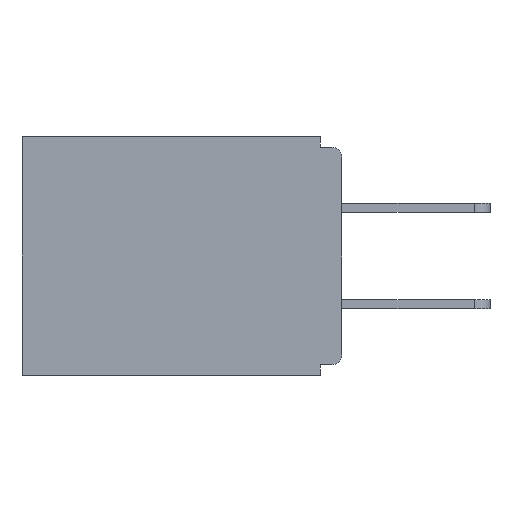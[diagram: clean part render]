
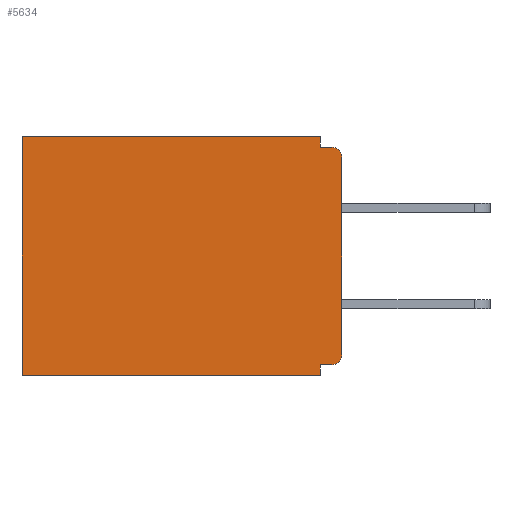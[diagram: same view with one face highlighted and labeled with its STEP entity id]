
A CAD part, left-side view. The second image highlights one B-rep face of the part: STEP entity #5634.
In plain terms, the highlighted planar face has unit normal (-1, 0, 0).
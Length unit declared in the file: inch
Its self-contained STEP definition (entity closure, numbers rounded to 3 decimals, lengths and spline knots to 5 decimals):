
#144 = VERTEX_POINT ( 'NONE', #15866 ) ;
#298 = VECTOR ( 'NONE', #16780, 39.37008 ) ;
#392 = DIRECTION ( 'NONE',  ( 0., 0., -1. ) ) ;
#428 = EDGE_CURVE ( 'NONE', #17263, #8227, #17666, .T. ) ;
#733 = ORIENTED_EDGE ( 'NONE', *, *, #4994, .F. ) ;
#946 = VECTOR ( 'NONE', #20086, 39.37008 ) ;
#1278 = CARTESIAN_POINT ( 'NONE',  ( 0.298, 0., -0.343 ) ) ;
#1414 = DIRECTION ( 'NONE',  ( -1., 0., 0. ) ) ;
#1761 = EDGE_CURVE ( 'NONE', #11068, #144, #8837, .T. ) ;
#1814 = VERTEX_POINT ( 'NONE', #16968 ) ;
#1829 = PLANE ( 'NONE',  #11761 ) ;
#2190 = DIRECTION ( 'NONE',  ( 0., 0., -1. ) ) ;
#3007 = DIRECTION ( 'NONE',  ( 0., 0., -1. ) ) ;
#3136 = CARTESIAN_POINT ( 'NONE',  ( 0.298, 0., 0. ) ) ;
#3260 = CARTESIAN_POINT ( 'NONE',  ( 0.298, 0.031, -0.343 ) ) ;
#3350 = CARTESIAN_POINT ( 'NONE',  ( 0.298, 0.031, -0.343 ) ) ;
#3386 = EDGE_CURVE ( 'NONE', #5225, #13934, #16574, .T. ) ;
#3631 = FACE_OUTER_BOUND ( 'NONE', #19337, .T. ) ;
#3820 = ORIENTED_EDGE ( 'NONE', *, *, #15078, .F. ) ;
#4227 = DIRECTION ( 'NONE',  ( 0., 0., -1. ) ) ;
#4338 = EDGE_CURVE ( 'NONE', #19054, #13934, #11926, .T. ) ;
#4565 = ORIENTED_EDGE ( 'NONE', *, *, #12514, .T. ) ;
#4671 = DIRECTION ( 'NONE',  ( 0., 1., 0. ) ) ;
#4994 = EDGE_CURVE ( 'NONE', #8227, #1814, #10667, .T. ) ;
#5121 = DIRECTION ( 'NONE',  ( 0., 0., -1. ) ) ;
#5212 = DIRECTION ( 'NONE',  ( -1., 0., 0. ) ) ;
#5225 = VERTEX_POINT ( 'NONE', #15585 ) ;
#5629 = ORIENTED_EDGE ( 'NONE', *, *, #3386, .T. ) ;
#5633 = VERTEX_POINT ( 'NONE', #14401 ) ;
#5634 = ADVANCED_FACE ( 'NONE', ( #3631 ), #1829, .F. ) ;
#5800 = CARTESIAN_POINT ( 'NONE',  ( 0.298, 0.031, -0.343 ) ) ;
#5917 = CARTESIAN_POINT ( 'NONE',  ( 0.298, 0.015, -0.03 ) ) ;
#5971 = LINE ( 'NONE', #20094, #12554 ) ;
#6472 = CARTESIAN_POINT ( 'NONE',  ( 0.298, 0., 0. ) ) ;
#6702 = CARTESIAN_POINT ( 'NONE',  ( 0.298, 0.031, -0.328 ) ) ;
#7814 = AXIS2_PLACEMENT_3D ( 'NONE', #8118, #5212, #2190 ) ;
#8021 = DIRECTION ( 'NONE',  ( 1., 0., 0. ) ) ;
#8118 = CARTESIAN_POINT ( 'NONE',  ( 0.298, 0.015, -0.313 ) ) ;
#8227 = VERTEX_POINT ( 'NONE', #3260 ) ;
#8309 = VERTEX_POINT ( 'NONE', #15780 ) ;
#8706 = VECTOR ( 'NONE', #9689, 39.37008 ) ;
#8831 = LINE ( 'NONE', #13582, #19780 ) ;
#8837 = LINE ( 'NONE', #3136, #20055 ) ;
#9355 = CARTESIAN_POINT ( 'NONE',  ( 0.298, 0., 0. ) ) ;
#9689 = DIRECTION ( 'NONE',  ( 0., 0., -1. ) ) ;
#10667 = LINE ( 'NONE', #1278, #298 ) ;
#11068 = VERTEX_POINT ( 'NONE', #14771 ) ;
#11761 = AXIS2_PLACEMENT_3D ( 'NONE', #6472, #8021, #5121 ) ;
#11926 = LINE ( 'NONE', #9355, #12911 ) ;
#12514 = EDGE_CURVE ( 'NONE', #144, #1814, #12669, .T. ) ;
#12554 = VECTOR ( 'NONE', #18431, 39.37008 ) ;
#12589 = ORIENTED_EDGE ( 'NONE', *, *, #1761, .T. ) ;
#12669 = LINE ( 'NONE', #16975, #19486 ) ;
#12911 = VECTOR ( 'NONE', #392, 39.37008 ) ;
#13455 = DIRECTION ( 'NONE',  ( 0., 1., 0. ) ) ;
#13582 = CARTESIAN_POINT ( 'NONE',  ( 0.298, 0., -0.328 ) ) ;
#13934 = VERTEX_POINT ( 'NONE', #18741 ) ;
#14060 = EDGE_CURVE ( 'NONE', #11068, #8309, #18420, .T. ) ;
#14282 = ORIENTED_EDGE ( 'NONE', *, *, #14060, .F. ) ;
#14401 = CARTESIAN_POINT ( 'NONE',  ( 0.298, 0.015, -0.015 ) ) ;
#14771 = CARTESIAN_POINT ( 'NONE',  ( 0.298, 0.031, 0. ) ) ;
#15078 = EDGE_CURVE ( 'NONE', #8309, #5633, #5971, .T. ) ;
#15585 = CARTESIAN_POINT ( 'NONE',  ( 0.298, 0.015, -0.328 ) ) ;
#15780 = CARTESIAN_POINT ( 'NONE',  ( 0.298, 0.031, -0.015 ) ) ;
#15866 = CARTESIAN_POINT ( 'NONE',  ( 0.298, 0.46, 0. ) ) ;
#16446 = CARTESIAN_POINT ( 'NONE',  ( 0.298, 0., -0.03 ) ) ;
#16574 = CIRCLE ( 'NONE', #7814, 0.015 ) ;
#16600 = CIRCLE ( 'NONE', #19985, 0.015 ) ;
#16780 = DIRECTION ( 'NONE',  ( 0., 1., 0. ) ) ;
#16968 = CARTESIAN_POINT ( 'NONE',  ( 0.298, 0.46, -0.343 ) ) ;
#16975 = CARTESIAN_POINT ( 'NONE',  ( 0.298, 0.46, 0. ) ) ;
#17263 = VERTEX_POINT ( 'NONE', #6702 ) ;
#17292 = ORIENTED_EDGE ( 'NONE', *, *, #4338, .F. ) ;
#17556 = EDGE_CURVE ( 'NONE', #19054, #5633, #16600, .T. ) ;
#17621 = ORIENTED_EDGE ( 'NONE', *, *, #428, .F. ) ;
#17666 = LINE ( 'NONE', #5800, #946 ) ;
#18420 = LINE ( 'NONE', #3350, #8706 ) ;
#18431 = DIRECTION ( 'NONE',  ( 0., -1., 0. ) ) ;
#18741 = CARTESIAN_POINT ( 'NONE',  ( 0.298, 0., -0.313 ) ) ;
#19054 = VERTEX_POINT ( 'NONE', #16446 ) ;
#19168 = EDGE_CURVE ( 'NONE', #5225, #17263, #8831, .T. ) ;
#19337 = EDGE_LOOP ( 'NONE', ( #20059, #3820, #14282, #12589, #4565, #733, #17621, #19573, #5629, #17292 ) ) ;
#19486 = VECTOR ( 'NONE', #3007, 39.37008 ) ;
#19573 = ORIENTED_EDGE ( 'NONE', *, *, #19168, .F. ) ;
#19780 = VECTOR ( 'NONE', #13455, 39.37008 ) ;
#19985 = AXIS2_PLACEMENT_3D ( 'NONE', #5917, #1414, #4227 ) ;
#20055 = VECTOR ( 'NONE', #4671, 39.37008 ) ;
#20059 = ORIENTED_EDGE ( 'NONE', *, *, #17556, .T. ) ;
#20086 = DIRECTION ( 'NONE',  ( 0., 0., -1. ) ) ;
#20094 = CARTESIAN_POINT ( 'NONE',  ( 0.298, 0., -0.015 ) ) ;
